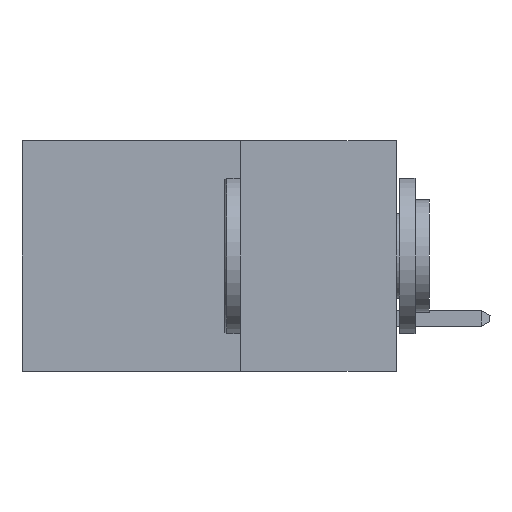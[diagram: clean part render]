
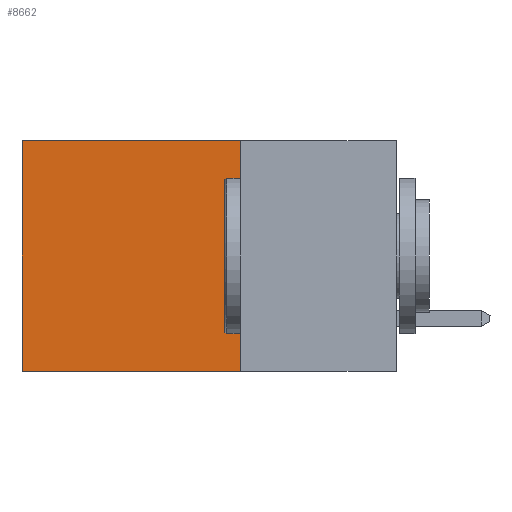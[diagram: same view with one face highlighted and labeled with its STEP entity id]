
A CAD part, left-side view. The second image highlights one B-rep face of the part: STEP entity #8662.
In plain terms, the highlighted planar face has unit normal (-1, 0, 0).
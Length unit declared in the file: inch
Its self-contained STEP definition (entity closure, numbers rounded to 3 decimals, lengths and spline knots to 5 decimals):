
#351 = CARTESIAN_POINT ( 'NONE',  ( 0.298, 0.25, -0.37 ) ) ;
#1514 = EDGE_CURVE ( 'NONE', #1698, #21509, #17645, .T. ) ;
#1698 = VERTEX_POINT ( 'NONE', #2140 ) ;
#2140 = CARTESIAN_POINT ( 'NONE',  ( 0.298, 0.6, 0. ) ) ;
#4249 = DIRECTION ( 'NONE',  ( 1., 0., 0. ) ) ;
#5924 = EDGE_LOOP ( 'NONE', ( #7598, #16783, #13173, #10724 ) ) ;
#5968 = LINE ( 'NONE', #23828, #14233 ) ;
#6567 = DIRECTION ( 'NONE',  ( 0., 0., -1. ) ) ;
#7598 = ORIENTED_EDGE ( 'NONE', *, *, #1514, .T. ) ;
#8515 = DIRECTION ( 'NONE',  ( 0., 0., -1. ) ) ;
#8662 = ADVANCED_FACE ( 'NONE', ( #24864 ), #28259, .F. ) ;
#9071 = CARTESIAN_POINT ( 'NONE',  ( 0.298, 0.6, 0. ) ) ;
#9777 = DIRECTION ( 'NONE',  ( 0., 1., 0. ) ) ;
#10181 = CARTESIAN_POINT ( 'NONE',  ( 0.298, 0.25, -0.37 ) ) ;
#10604 = VECTOR ( 'NONE', #8515, 39.37008 ) ;
#10724 = ORIENTED_EDGE ( 'NONE', *, *, #13730, .T. ) ;
#13173 = ORIENTED_EDGE ( 'NONE', *, *, #27627, .F. ) ;
#13178 = VECTOR ( 'NONE', #9777, 39.37008 ) ;
#13730 = EDGE_CURVE ( 'NONE', #28245, #1698, #5968, .T. ) ;
#13864 = CARTESIAN_POINT ( 'NONE',  ( 0.298, 0.25, 0. ) ) ;
#14233 = VECTOR ( 'NONE', #23616, 39.37008 ) ;
#16203 = LINE ( 'NONE', #351, #13178 ) ;
#16783 = ORIENTED_EDGE ( 'NONE', *, *, #29975, .F. ) ;
#17220 = CARTESIAN_POINT ( 'NONE',  ( 0.298, 0.6, -0.37 ) ) ;
#17645 = LINE ( 'NONE', #9071, #25869 ) ;
#20337 = VERTEX_POINT ( 'NONE', #10181 ) ;
#20791 = CARTESIAN_POINT ( 'NONE',  ( 0.298, 0.25, 0. ) ) ;
#21110 = DIRECTION ( 'NONE',  ( 0., 0., -1. ) ) ;
#21509 = VERTEX_POINT ( 'NONE', #17220 ) ;
#23616 = DIRECTION ( 'NONE',  ( 0., 1., 0. ) ) ;
#23759 = AXIS2_PLACEMENT_3D ( 'NONE', #13864, #4249, #21110 ) ;
#23828 = CARTESIAN_POINT ( 'NONE',  ( 0.298, 0.25, 0. ) ) ;
#24864 = FACE_OUTER_BOUND ( 'NONE', #5924, .T. ) ;
#25335 = CARTESIAN_POINT ( 'NONE',  ( 0.298, 0.25, 0. ) ) ;
#25869 = VECTOR ( 'NONE', #6567, 39.37008 ) ;
#27627 = EDGE_CURVE ( 'NONE', #28245, #20337, #28679, .T. ) ;
#28245 = VERTEX_POINT ( 'NONE', #20791 ) ;
#28259 = PLANE ( 'NONE',  #23759 ) ;
#28679 = LINE ( 'NONE', #25335, #10604 ) ;
#29975 = EDGE_CURVE ( 'NONE', #20337, #21509, #16203, .T. ) ;
